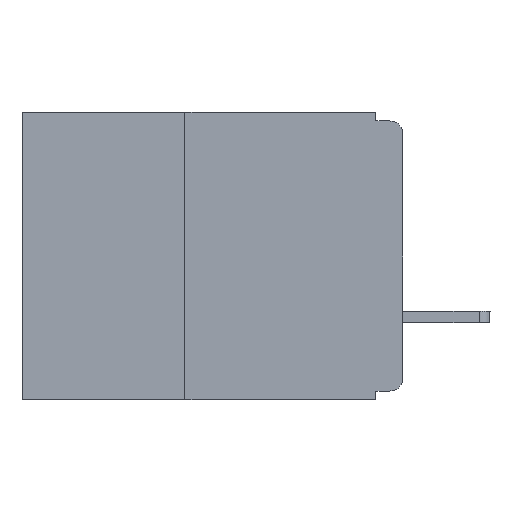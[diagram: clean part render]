
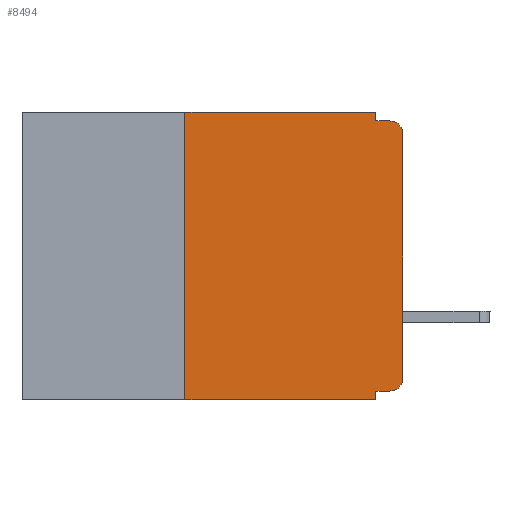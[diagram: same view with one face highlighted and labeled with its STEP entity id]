
A CAD part, left-side view. The second image highlights one B-rep face of the part: STEP entity #8494.
In plain terms, the highlighted planar face has unit normal (-1, 0, 0).
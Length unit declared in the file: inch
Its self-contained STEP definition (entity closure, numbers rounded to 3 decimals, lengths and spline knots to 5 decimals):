
#400 = VERTEX_POINT ( 'NONE', #8760 ) ;
#413 = VERTEX_POINT ( 'NONE', #1178 ) ;
#424 = ORIENTED_EDGE ( 'NONE', *, *, #937, .F. ) ;
#648 = VERTEX_POINT ( 'NONE', #2574 ) ;
#650 = LINE ( 'NONE', #11706, #1671 ) ;
#728 = VERTEX_POINT ( 'NONE', #4017 ) ;
#879 = LINE ( 'NONE', #14193, #6049 ) ;
#937 = EDGE_CURVE ( 'NONE', #7306, #4951, #879, .T. ) ;
#1178 = CARTESIAN_POINT ( 'NONE',  ( 0., 0., -0.025 ) ) ;
#1448 = CARTESIAN_POINT ( 'NONE',  ( 0., 0.25, -0.33 ) ) ;
#1671 = VECTOR ( 'NONE', #12988, 39.37008 ) ;
#1768 = VECTOR ( 'NONE', #12462, 39.37008 ) ;
#1889 = VECTOR ( 'NONE', #12770, 39.37008 ) ;
#1919 = AXIS2_PLACEMENT_3D ( 'NONE', #9106, #4666, #5763 ) ;
#2057 = VECTOR ( 'NONE', #14108, 39.37008 ) ;
#2161 = CIRCLE ( 'NONE', #5650, 0.015 ) ;
#2574 = CARTESIAN_POINT ( 'NONE',  ( 0., 0.031, -0.01 ) ) ;
#2713 = VERTEX_POINT ( 'NONE', #10028 ) ;
#3030 = ORIENTED_EDGE ( 'NONE', *, *, #7970, .F. ) ;
#3282 = DIRECTION ( 'NONE',  ( 1., 0., 0. ) ) ;
#3375 = PLANE ( 'NONE',  #12070 ) ;
#3408 = VERTEX_POINT ( 'NONE', #4979 ) ;
#3496 = CARTESIAN_POINT ( 'NONE',  ( 0., 0.031, -0.33 ) ) ;
#3765 = FACE_OUTER_BOUND ( 'NONE', #11633, .T. ) ;
#3967 = LINE ( 'NONE', #11655, #1889 ) ;
#4017 = CARTESIAN_POINT ( 'NONE',  ( 0., 0.015, -0.01 ) ) ;
#4065 = ORIENTED_EDGE ( 'NONE', *, *, #5070, .T. ) ;
#4406 = EDGE_CURVE ( 'NONE', #3408, #413, #12937, .T. ) ;
#4470 = CARTESIAN_POINT ( 'NONE',  ( 0., 0.015, -0.305 ) ) ;
#4666 = DIRECTION ( 'NONE',  ( -1., 0., 0. ) ) ;
#4682 = CARTESIAN_POINT ( 'NONE',  ( 0., 0.25, 0. ) ) ;
#4723 = LINE ( 'NONE', #1448, #1768 ) ;
#4951 = VERTEX_POINT ( 'NONE', #6638 ) ;
#4979 = CARTESIAN_POINT ( 'NONE',  ( 0., 0., -0.305 ) ) ;
#5070 = EDGE_CURVE ( 'NONE', #2713, #3408, #2161, .T. ) ;
#5650 = AXIS2_PLACEMENT_3D ( 'NONE', #4470, #13331, #6685 ) ;
#5763 = DIRECTION ( 'NONE',  ( 0., 0., -1. ) ) ;
#6049 = VECTOR ( 'NONE', #7475, 39.37008 ) ;
#6592 = CARTESIAN_POINT ( 'NONE',  ( 0., 0.437, 0. ) ) ;
#6638 = CARTESIAN_POINT ( 'NONE',  ( 0., 0.031, 0. ) ) ;
#6685 = DIRECTION ( 'NONE',  ( 0., 0., -1. ) ) ;
#6880 = ORIENTED_EDGE ( 'NONE', *, *, #7177, .F. ) ;
#7005 = ORIENTED_EDGE ( 'NONE', *, *, #7705, .T. ) ;
#7009 = EDGE_CURVE ( 'NONE', #400, #13838, #3967, .T. ) ;
#7177 = EDGE_CURVE ( 'NONE', #648, #728, #13840, .T. ) ;
#7229 = DIRECTION ( 'NONE',  ( 0., 0., 1. ) ) ;
#7306 = VERTEX_POINT ( 'NONE', #4682 ) ;
#7472 = LINE ( 'NONE', #10672, #9917 ) ;
#7475 = DIRECTION ( 'NONE',  ( 0., -1., 0. ) ) ;
#7685 = ORIENTED_EDGE ( 'NONE', *, *, #9102, .F. ) ;
#7705 = EDGE_CURVE ( 'NONE', #413, #728, #8780, .T. ) ;
#7970 = EDGE_CURVE ( 'NONE', #4951, #648, #650, .T. ) ;
#7991 = ORIENTED_EDGE ( 'NONE', *, *, #4406, .T. ) ;
#8277 = ORIENTED_EDGE ( 'NONE', *, *, #13910, .F. ) ;
#8494 = ADVANCED_FACE ( 'NONE', ( #3765 ), #3375, .F. ) ;
#8501 = ORIENTED_EDGE ( 'NONE', *, *, #10738, .F. ) ;
#8760 = CARTESIAN_POINT ( 'NONE',  ( 0., 0.25, -0.33 ) ) ;
#8780 = CIRCLE ( 'NONE', #1919, 0.015 ) ;
#8814 = DIRECTION ( 'NONE',  ( 0., 0., -1. ) ) ;
#9102 = EDGE_CURVE ( 'NONE', #11884, #13838, #12578, .T. ) ;
#9106 = CARTESIAN_POINT ( 'NONE',  ( 0., 0.015, -0.025 ) ) ;
#9295 = CARTESIAN_POINT ( 'NONE',  ( 0., 0.031, -0.32 ) ) ;
#9917 = VECTOR ( 'NONE', #11648, 39.37008 ) ;
#10028 = CARTESIAN_POINT ( 'NONE',  ( 0., 0.015, -0.32 ) ) ;
#10672 = CARTESIAN_POINT ( 'NONE',  ( 0., 0., -0.32 ) ) ;
#10738 = EDGE_CURVE ( 'NONE', #2713, #11884, #7472, .T. ) ;
#10869 = CARTESIAN_POINT ( 'NONE',  ( 0., 0., -0.01 ) ) ;
#11395 = ORIENTED_EDGE ( 'NONE', *, *, #7009, .T. ) ;
#11633 = EDGE_LOOP ( 'NONE', ( #7991, #7005, #6880, #3030, #424, #8277, #11395, #7685, #8501, #4065 ) ) ;
#11648 = DIRECTION ( 'NONE',  ( 0., 1., 0. ) ) ;
#11655 = CARTESIAN_POINT ( 'NONE',  ( 0., 0.437, -0.33 ) ) ;
#11706 = CARTESIAN_POINT ( 'NONE',  ( 0., 0.031, 0. ) ) ;
#11884 = VERTEX_POINT ( 'NONE', #9295 ) ;
#12070 = AXIS2_PLACEMENT_3D ( 'NONE', #6592, #3282, #13154 ) ;
#12080 = VECTOR ( 'NONE', #8814, 39.37008 ) ;
#12462 = DIRECTION ( 'NONE',  ( 0., 0., 1. ) ) ;
#12578 = LINE ( 'NONE', #13340, #12080 ) ;
#12590 = VECTOR ( 'NONE', #7229, 39.37008 ) ;
#12770 = DIRECTION ( 'NONE',  ( 0., -1., 0. ) ) ;
#12937 = LINE ( 'NONE', #13015, #12590 ) ;
#12988 = DIRECTION ( 'NONE',  ( 0., 0., -1. ) ) ;
#13015 = CARTESIAN_POINT ( 'NONE',  ( 0., 0., 0. ) ) ;
#13154 = DIRECTION ( 'NONE',  ( 0., 0., -1. ) ) ;
#13331 = DIRECTION ( 'NONE',  ( -1., 0., 0. ) ) ;
#13340 = CARTESIAN_POINT ( 'NONE',  ( 0., 0.031, -0.33 ) ) ;
#13838 = VERTEX_POINT ( 'NONE', #3496 ) ;
#13840 = LINE ( 'NONE', #10869, #2057 ) ;
#13910 = EDGE_CURVE ( 'NONE', #400, #7306, #4723, .T. ) ;
#14108 = DIRECTION ( 'NONE',  ( 0., -1., 0. ) ) ;
#14193 = CARTESIAN_POINT ( 'NONE',  ( 0., 0.437, 0. ) ) ;
